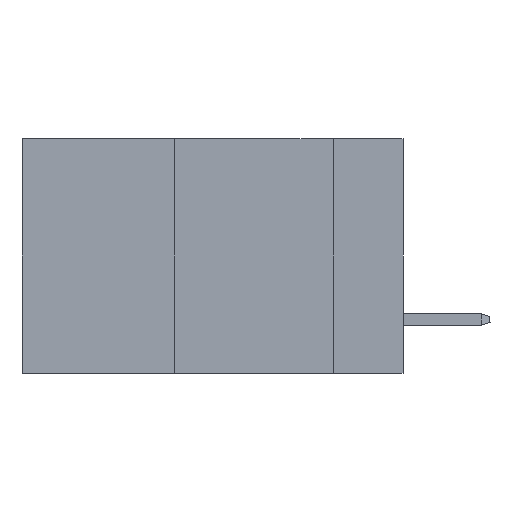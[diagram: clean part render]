
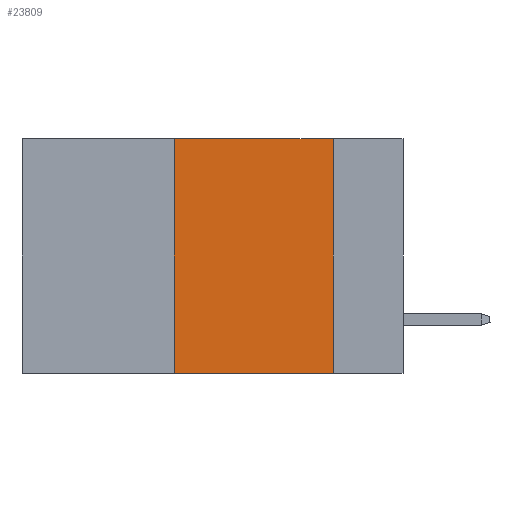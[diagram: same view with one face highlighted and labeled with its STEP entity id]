
A CAD part, left-side view. The second image highlights one B-rep face of the part: STEP entity #23809.
In plain terms, the highlighted planar face has unit normal (-1, 0, 0).
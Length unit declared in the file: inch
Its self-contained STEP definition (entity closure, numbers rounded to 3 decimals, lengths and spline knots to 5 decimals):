
#391 = ORIENTED_EDGE ( 'NONE', *, *, #28194, .T. ) ;
#939 = LINE ( 'NONE', #29370, #31083 ) ;
#1467 = VECTOR ( 'NONE', #17125, 39.37008 ) ;
#1590 = DIRECTION ( 'NONE',  ( 0., 0., -1. ) ) ;
#2405 = VECTOR ( 'NONE', #21454, 39.37008 ) ;
#3976 = EDGE_CURVE ( 'NONE', #7794, #15993, #939, .T. ) ;
#6761 = CARTESIAN_POINT ( 'NONE',  ( 0., 0.11, 0. ) ) ;
#7794 = VERTEX_POINT ( 'NONE', #6761 ) ;
#7974 = EDGE_CURVE ( 'NONE', #17148, #28846, #10147, .T. ) ;
#8548 = CARTESIAN_POINT ( 'NONE',  ( 0., 0.6, -0.37 ) ) ;
#9947 = FACE_OUTER_BOUND ( 'NONE', #17617, .T. ) ;
#10147 = LINE ( 'NONE', #28018, #1467 ) ;
#15607 = AXIS2_PLACEMENT_3D ( 'NONE', #24941, #27658, #1590 ) ;
#15993 = VERTEX_POINT ( 'NONE', #17935 ) ;
#17125 = DIRECTION ( 'NONE',  ( 0., 0., 1. ) ) ;
#17148 = VERTEX_POINT ( 'NONE', #20549 ) ;
#17617 = EDGE_LOOP ( 'NONE', ( #24383, #31203, #19586, #391 ) ) ;
#17935 = CARTESIAN_POINT ( 'NONE',  ( 0., 0.11, -0.37 ) ) ;
#19586 = ORIENTED_EDGE ( 'NONE', *, *, #7974, .F. ) ;
#20549 = CARTESIAN_POINT ( 'NONE',  ( 0., 0.36, -0.37 ) ) ;
#21454 = DIRECTION ( 'NONE',  ( 0., -1., 0. ) ) ;
#23280 = DIRECTION ( 'NONE',  ( 0., -1., 0. ) ) ;
#23809 = ADVANCED_FACE ( 'NONE', ( #9947 ), #27978, .F. ) ;
#24383 = ORIENTED_EDGE ( 'NONE', *, *, #3976, .F. ) ;
#24772 = DIRECTION ( 'NONE',  ( 0., 0., -1. ) ) ;
#24941 = CARTESIAN_POINT ( 'NONE',  ( 0., 0.6, 0. ) ) ;
#25346 = CARTESIAN_POINT ( 'NONE',  ( 0., 0.6, 0. ) ) ;
#26009 = VECTOR ( 'NONE', #23280, 39.37008 ) ;
#27658 = DIRECTION ( 'NONE',  ( 1., 0., 0. ) ) ;
#27978 = PLANE ( 'NONE',  #15607 ) ;
#28018 = CARTESIAN_POINT ( 'NONE',  ( 0., 0.36, 0. ) ) ;
#28194 = EDGE_CURVE ( 'NONE', #17148, #15993, #32521, .T. ) ;
#28846 = VERTEX_POINT ( 'NONE', #28998 ) ;
#28998 = CARTESIAN_POINT ( 'NONE',  ( 0., 0.36, 0. ) ) ;
#29370 = CARTESIAN_POINT ( 'NONE',  ( 0., 0.11, 0. ) ) ;
#30791 = LINE ( 'NONE', #25346, #26009 ) ;
#31083 = VECTOR ( 'NONE', #24772, 39.37008 ) ;
#31203 = ORIENTED_EDGE ( 'NONE', *, *, #32253, .F. ) ;
#32253 = EDGE_CURVE ( 'NONE', #28846, #7794, #30791, .T. ) ;
#32521 = LINE ( 'NONE', #8548, #2405 ) ;
